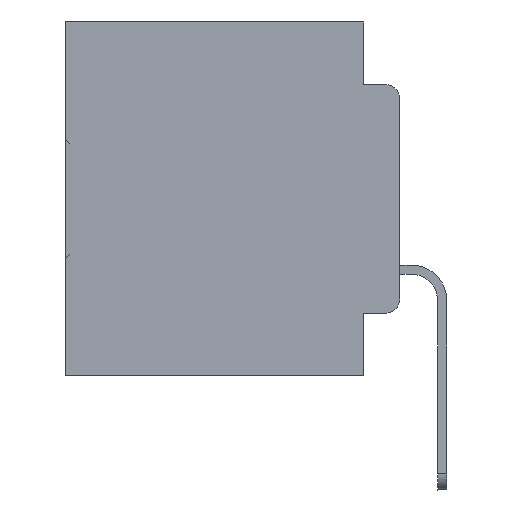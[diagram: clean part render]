
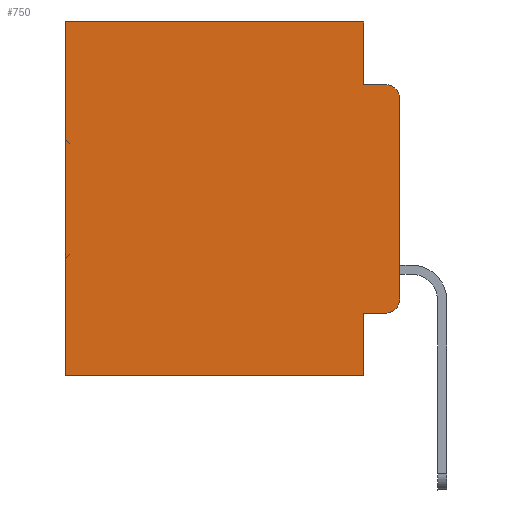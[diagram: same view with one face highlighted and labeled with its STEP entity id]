
A CAD part, left-side view. The second image highlights one B-rep face of the part: STEP entity #750.
In plain terms, the highlighted planar face has unit normal (-1, 0, 0).
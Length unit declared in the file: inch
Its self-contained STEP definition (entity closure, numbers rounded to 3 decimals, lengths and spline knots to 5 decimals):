
#678 = EDGE_CURVE ( 'NONE', #28471, #4563, #6746, .T. ) ;
#750 = ADVANCED_FACE ( 'NONE', ( #15628 ), #29186, .F. ) ;
#918 = EDGE_CURVE ( 'NONE', #28471, #1659, #3418, .T. ) ;
#993 = EDGE_CURVE ( 'NONE', #16408, #1659, #4951, .T. ) ;
#1659 = VERTEX_POINT ( 'NONE', #20951 ) ;
#1771 = EDGE_CURVE ( 'NONE', #20927, #9840, #26497, .T. ) ;
#3060 = ORIENTED_EDGE ( 'NONE', *, *, #29624, .T. ) ;
#3355 = VERTEX_POINT ( 'NONE', #18232 ) ;
#3416 = AXIS2_PLACEMENT_3D ( 'NONE', #11676, #24719, #9070 ) ;
#3418 = LINE ( 'NONE', #30009, #4378 ) ;
#3507 = CARTESIAN_POINT ( 'NONE',  ( 0.298, 0., -0.1085 ) ) ;
#3780 = EDGE_CURVE ( 'NONE', #9840, #12040, #21262, .T. ) ;
#3922 = DIRECTION ( 'NONE',  ( 0., 0., -1. ) ) ;
#4155 = ORIENTED_EDGE ( 'NONE', *, *, #918, .F. ) ;
#4202 = DIRECTION ( 'NONE',  ( 1., 0., 0. ) ) ;
#4378 = VECTOR ( 'NONE', #26733, 39.37008 ) ;
#4503 = DIRECTION ( 'NONE',  ( 0., 1., 0. ) ) ;
#4563 = VERTEX_POINT ( 'NONE', #8836 ) ;
#4951 = CIRCLE ( 'NONE', #21603, 0.02 ) ;
#5059 = CARTESIAN_POINT ( 'NONE',  ( 0.298, 0.051, -0.0885 ) ) ;
#5186 = DIRECTION ( 'NONE',  ( 0., 0., -1. ) ) ;
#5685 = CARTESIAN_POINT ( 'NONE',  ( 0.298, 0.051, 0. ) ) ;
#6015 = VERTEX_POINT ( 'NONE', #5685 ) ;
#6746 = CIRCLE ( 'NONE', #3416, 0.02 ) ;
#7353 = DIRECTION ( 'NONE',  ( 0., 1., 0. ) ) ;
#7557 = VECTOR ( 'NONE', #21146, 39.37008 ) ;
#8801 = CARTESIAN_POINT ( 'NONE',  ( 0.298, 0.051, -0.5 ) ) ;
#8836 = CARTESIAN_POINT ( 'NONE',  ( 0.298, 0.02, -0.0885 ) ) ;
#9070 = DIRECTION ( 'NONE',  ( 0., 0., -1. ) ) ;
#9104 = LINE ( 'NONE', #9279, #29457 ) ;
#9279 = CARTESIAN_POINT ( 'NONE',  ( 0.298, 0.051, 0. ) ) ;
#9323 = ORIENTED_EDGE ( 'NONE', *, *, #3780, .F. ) ;
#9840 = VERTEX_POINT ( 'NONE', #8801 ) ;
#10201 = CARTESIAN_POINT ( 'NONE',  ( 0.298, 0.051, -0.4115 ) ) ;
#10662 = CARTESIAN_POINT ( 'NONE',  ( 0.298, 0.051, 0. ) ) ;
#11647 = VERTEX_POINT ( 'NONE', #20792 ) ;
#11676 = CARTESIAN_POINT ( 'NONE',  ( 0.298, 0.02, -0.1085 ) ) ;
#11949 = CARTESIAN_POINT ( 'NONE',  ( 0.298, 0.02, -0.3915 ) ) ;
#12040 = VERTEX_POINT ( 'NONE', #30470 ) ;
#12216 = VECTOR ( 'NONE', #18502, 39.37008 ) ;
#14484 = EDGE_CURVE ( 'NONE', #6015, #11647, #9104, .T. ) ;
#14797 = ORIENTED_EDGE ( 'NONE', *, *, #23708, .T. ) ;
#15124 = LINE ( 'NONE', #17734, #21832 ) ;
#15212 = VECTOR ( 'NONE', #7353, 39.37008 ) ;
#15434 = ORIENTED_EDGE ( 'NONE', *, *, #16576, .T. ) ;
#15628 = FACE_OUTER_BOUND ( 'NONE', #18842, .T. ) ;
#15980 = CARTESIAN_POINT ( 'NONE',  ( 0.298, 0., 0. ) ) ;
#16115 = EDGE_CURVE ( 'NONE', #11647, #4563, #26103, .T. ) ;
#16408 = VERTEX_POINT ( 'NONE', #31995 ) ;
#16479 = VECTOR ( 'NONE', #31906, 39.37008 ) ;
#16576 = EDGE_CURVE ( 'NONE', #6015, #3355, #15124, .T. ) ;
#17117 = DIRECTION ( 'NONE',  ( 0., 0., -1. ) ) ;
#17734 = CARTESIAN_POINT ( 'NONE',  ( 0.298, 0., 0. ) ) ;
#18200 = CARTESIAN_POINT ( 'NONE',  ( 0.298, 0.473, 0. ) ) ;
#18232 = CARTESIAN_POINT ( 'NONE',  ( 0.298, 0.473, 0. ) ) ;
#18502 = DIRECTION ( 'NONE',  ( 0., 0., -1. ) ) ;
#18842 = EDGE_LOOP ( 'NONE', ( #4155, #28053, #20937, #31046, #15434, #14797, #9323, #33682, #3060, #29159 ) ) ;
#20088 = AXIS2_PLACEMENT_3D ( 'NONE', #15980, #4202, #5186 ) ;
#20792 = CARTESIAN_POINT ( 'NONE',  ( 0.298, 0.051, -0.0885 ) ) ;
#20927 = VERTEX_POINT ( 'NONE', #33684 ) ;
#20937 = ORIENTED_EDGE ( 'NONE', *, *, #16115, .F. ) ;
#20951 = CARTESIAN_POINT ( 'NONE',  ( 0.298, 0., -0.3915 ) ) ;
#21146 = DIRECTION ( 'NONE',  ( 0., -1., 0. ) ) ;
#21262 = LINE ( 'NONE', #23528, #15212 ) ;
#21603 = AXIS2_PLACEMENT_3D ( 'NONE', #11949, #30528, #3922 ) ;
#21832 = VECTOR ( 'NONE', #4503, 39.37008 ) ;
#22931 = VECTOR ( 'NONE', #31136, 39.37008 ) ;
#23528 = CARTESIAN_POINT ( 'NONE',  ( 0.298, 0., -0.5 ) ) ;
#23583 = LINE ( 'NONE', #18200, #16479 ) ;
#23708 = EDGE_CURVE ( 'NONE', #3355, #12040, #23583, .T. ) ;
#24719 = DIRECTION ( 'NONE',  ( -1., 0., 0. ) ) ;
#26103 = LINE ( 'NONE', #5059, #22931 ) ;
#26497 = LINE ( 'NONE', #10662, #12216 ) ;
#26733 = DIRECTION ( 'NONE',  ( 0., 0., -1. ) ) ;
#28053 = ORIENTED_EDGE ( 'NONE', *, *, #678, .T. ) ;
#28471 = VERTEX_POINT ( 'NONE', #3507 ) ;
#29159 = ORIENTED_EDGE ( 'NONE', *, *, #993, .T. ) ;
#29186 = PLANE ( 'NONE',  #20088 ) ;
#29457 = VECTOR ( 'NONE', #17117, 39.37008 ) ;
#29624 = EDGE_CURVE ( 'NONE', #20927, #16408, #31914, .T. ) ;
#30009 = CARTESIAN_POINT ( 'NONE',  ( 0.298, 0., 0. ) ) ;
#30470 = CARTESIAN_POINT ( 'NONE',  ( 0.298, 0.473, -0.5 ) ) ;
#30528 = DIRECTION ( 'NONE',  ( -1., 0., 0. ) ) ;
#31046 = ORIENTED_EDGE ( 'NONE', *, *, #14484, .F. ) ;
#31136 = DIRECTION ( 'NONE',  ( 0., -1., 0. ) ) ;
#31906 = DIRECTION ( 'NONE',  ( 0., 0., -1. ) ) ;
#31914 = LINE ( 'NONE', #10201, #7557 ) ;
#31995 = CARTESIAN_POINT ( 'NONE',  ( 0.298, 0.02, -0.4115 ) ) ;
#33682 = ORIENTED_EDGE ( 'NONE', *, *, #1771, .F. ) ;
#33684 = CARTESIAN_POINT ( 'NONE',  ( 0.298, 0.051, -0.4115 ) ) ;
